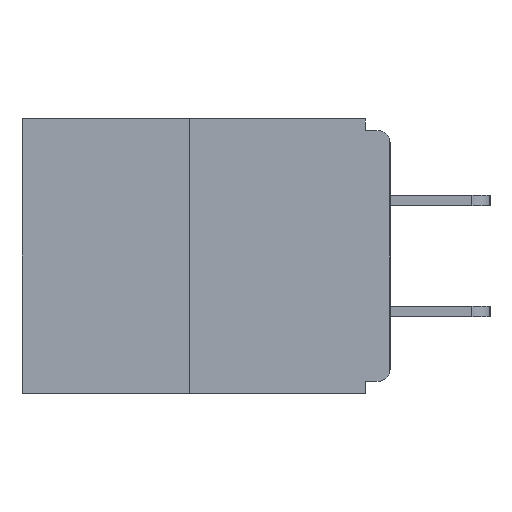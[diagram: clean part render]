
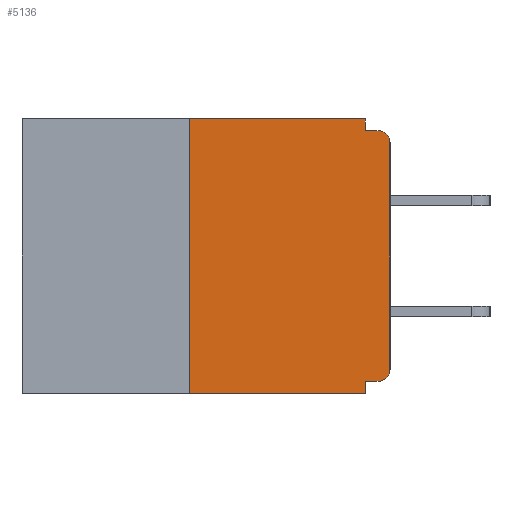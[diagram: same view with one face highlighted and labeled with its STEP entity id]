
A CAD part, left-side view. The second image highlights one B-rep face of the part: STEP entity #5136.
In plain terms, the highlighted planar face has unit normal (-1, 0, 0).
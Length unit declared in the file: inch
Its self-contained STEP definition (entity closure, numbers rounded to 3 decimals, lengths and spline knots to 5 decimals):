
#122 = ORIENTED_EDGE ( 'NONE', *, *, #3043, .T. ) ;
#365 = CARTESIAN_POINT ( 'NONE',  ( 0., 0.015, -0.03 ) ) ;
#833 = CIRCLE ( 'NONE', #8427, 0.015 ) ;
#1061 = DIRECTION ( 'NONE',  ( 1., 0., 0. ) ) ;
#1106 = FACE_OUTER_BOUND ( 'NONE', #1296, .T. ) ;
#1296 = EDGE_LOOP ( 'NONE', ( #7498, #6534, #122, #7452, #13920, #4555, #16134, #4345, #12103, #6657 ) ) ;
#1421 = CARTESIAN_POINT ( 'NONE',  ( 0., 0.031, -0.328 ) ) ;
#1895 = EDGE_CURVE ( 'NONE', #16887, #13287, #833, .T. ) ;
#2013 = AXIS2_PLACEMENT_3D ( 'NONE', #17414, #1061, #11947 ) ;
#2375 = CARTESIAN_POINT ( 'NONE',  ( 0., 0.25, 0. ) ) ;
#2618 = CARTESIAN_POINT ( 'NONE',  ( 0., 0.015, -0.015 ) ) ;
#2912 = EDGE_CURVE ( 'NONE', #16887, #11856, #6688, .T. ) ;
#3043 = EDGE_CURVE ( 'NONE', #8621, #14636, #8831, .T. ) ;
#3685 = CARTESIAN_POINT ( 'NONE',  ( 0., 0.46, 0. ) ) ;
#4121 = DIRECTION ( 'NONE',  ( 0., 0., -1. ) ) ;
#4256 = EDGE_CURVE ( 'NONE', #6105, #15358, #7068, .T. ) ;
#4345 = ORIENTED_EDGE ( 'NONE', *, *, #5379, .T. ) ;
#4555 = ORIENTED_EDGE ( 'NONE', *, *, #1895, .T. ) ;
#4605 = LINE ( 'NONE', #3685, #12674 ) ;
#4771 = LINE ( 'NONE', #16343, #8136 ) ;
#4880 = CARTESIAN_POINT ( 'NONE',  ( 0., 0., 0. ) ) ;
#5120 = PLANE ( 'NONE',  #2013 ) ;
#5136 = ADVANCED_FACE ( 'NONE', ( #1106 ), #5120, .F. ) ;
#5161 = VECTOR ( 'NONE', #4121, 39.37008 ) ;
#5211 = VECTOR ( 'NONE', #15594, 39.37008 ) ;
#5226 = CARTESIAN_POINT ( 'NONE',  ( 0., 0.031, 0. ) ) ;
#5379 = EDGE_CURVE ( 'NONE', #6828, #13821, #17358, .T. ) ;
#5788 = VECTOR ( 'NONE', #17113, 39.37008 ) ;
#5861 = AXIS2_PLACEMENT_3D ( 'NONE', #365, #11227, #9800 ) ;
#5937 = CARTESIAN_POINT ( 'NONE',  ( 0., 0., -0.313 ) ) ;
#6105 = VERTEX_POINT ( 'NONE', #12502 ) ;
#6534 = ORIENTED_EDGE ( 'NONE', *, *, #10065, .F. ) ;
#6657 = ORIENTED_EDGE ( 'NONE', *, *, #4256, .F. ) ;
#6688 = LINE ( 'NONE', #9860, #9040 ) ;
#6828 = VERTEX_POINT ( 'NONE', #15173 ) ;
#6889 = DIRECTION ( 'NONE',  ( 0., -1., 0. ) ) ;
#7068 = LINE ( 'NONE', #5226, #5161 ) ;
#7412 = CARTESIAN_POINT ( 'NONE',  ( 0., 0.46, -0.343 ) ) ;
#7452 = ORIENTED_EDGE ( 'NONE', *, *, #9383, .F. ) ;
#7498 = ORIENTED_EDGE ( 'NONE', *, *, #16519, .F. ) ;
#8136 = VECTOR ( 'NONE', #11333, 39.37008 ) ;
#8427 = AXIS2_PLACEMENT_3D ( 'NONE', #13132, #17126, #8851 ) ;
#8621 = VERTEX_POINT ( 'NONE', #10457 ) ;
#8831 = LINE ( 'NONE', #7412, #5211 ) ;
#8851 = DIRECTION ( 'NONE',  ( 0., 0., -1. ) ) ;
#8912 = CARTESIAN_POINT ( 'NONE',  ( 0., 0.031, -0.343 ) ) ;
#8929 = CARTESIAN_POINT ( 'NONE',  ( 0., 0.015, -0.328 ) ) ;
#9040 = VECTOR ( 'NONE', #12653, 39.37008 ) ;
#9383 = EDGE_CURVE ( 'NONE', #11856, #14636, #4771, .T. ) ;
#9729 = DIRECTION ( 'NONE',  ( 0., 0., 1. ) ) ;
#9800 = DIRECTION ( 'NONE',  ( 0., 0., -1. ) ) ;
#9860 = CARTESIAN_POINT ( 'NONE',  ( 0., 0., -0.328 ) ) ;
#10065 = EDGE_CURVE ( 'NONE', #8621, #15101, #13645, .T. ) ;
#10457 = CARTESIAN_POINT ( 'NONE',  ( 0., 0.25, -0.343 ) ) ;
#10598 = EDGE_CURVE ( 'NONE', #15358, #13821, #13631, .T. ) ;
#11227 = DIRECTION ( 'NONE',  ( -1., 0., 0. ) ) ;
#11299 = VECTOR ( 'NONE', #6889, 39.37008 ) ;
#11333 = DIRECTION ( 'NONE',  ( 0., 0., -1. ) ) ;
#11856 = VERTEX_POINT ( 'NONE', #1421 ) ;
#11944 = VECTOR ( 'NONE', #9729, 39.37008 ) ;
#11947 = DIRECTION ( 'NONE',  ( 0., 0., -1. ) ) ;
#12103 = ORIENTED_EDGE ( 'NONE', *, *, #10598, .F. ) ;
#12311 = EDGE_CURVE ( 'NONE', #13287, #6828, #16371, .T. ) ;
#12502 = CARTESIAN_POINT ( 'NONE',  ( 0., 0.031, 0. ) ) ;
#12653 = DIRECTION ( 'NONE',  ( 0., 1., 0. ) ) ;
#12674 = VECTOR ( 'NONE', #17224, 39.37008 ) ;
#13132 = CARTESIAN_POINT ( 'NONE',  ( 0., 0.015, -0.313 ) ) ;
#13287 = VERTEX_POINT ( 'NONE', #5937 ) ;
#13631 = LINE ( 'NONE', #16252, #11299 ) ;
#13645 = LINE ( 'NONE', #15108, #11944 ) ;
#13821 = VERTEX_POINT ( 'NONE', #2618 ) ;
#13920 = ORIENTED_EDGE ( 'NONE', *, *, #2912, .F. ) ;
#14103 = CARTESIAN_POINT ( 'NONE',  ( 0., 0.031, -0.015 ) ) ;
#14636 = VERTEX_POINT ( 'NONE', #8912 ) ;
#15101 = VERTEX_POINT ( 'NONE', #2375 ) ;
#15108 = CARTESIAN_POINT ( 'NONE',  ( 0., 0.25, 0. ) ) ;
#15173 = CARTESIAN_POINT ( 'NONE',  ( 0., 0., -0.03 ) ) ;
#15358 = VERTEX_POINT ( 'NONE', #14103 ) ;
#15594 = DIRECTION ( 'NONE',  ( 0., -1., 0. ) ) ;
#16134 = ORIENTED_EDGE ( 'NONE', *, *, #12311, .T. ) ;
#16252 = CARTESIAN_POINT ( 'NONE',  ( 0., 0., -0.015 ) ) ;
#16343 = CARTESIAN_POINT ( 'NONE',  ( 0., 0.031, -0.343 ) ) ;
#16371 = LINE ( 'NONE', #4880, #5788 ) ;
#16519 = EDGE_CURVE ( 'NONE', #15101, #6105, #4605, .T. ) ;
#16887 = VERTEX_POINT ( 'NONE', #8929 ) ;
#17113 = DIRECTION ( 'NONE',  ( 0., 0., 1. ) ) ;
#17126 = DIRECTION ( 'NONE',  ( -1., 0., 0. ) ) ;
#17224 = DIRECTION ( 'NONE',  ( 0., -1., 0. ) ) ;
#17358 = CIRCLE ( 'NONE', #5861, 0.015 ) ;
#17414 = CARTESIAN_POINT ( 'NONE',  ( 0., 0.46, 0. ) ) ;
